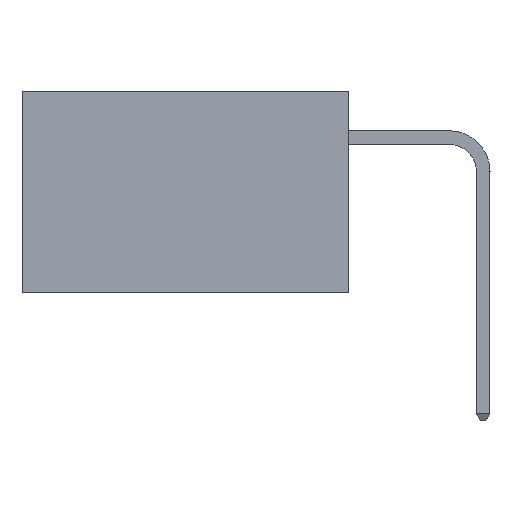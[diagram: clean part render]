
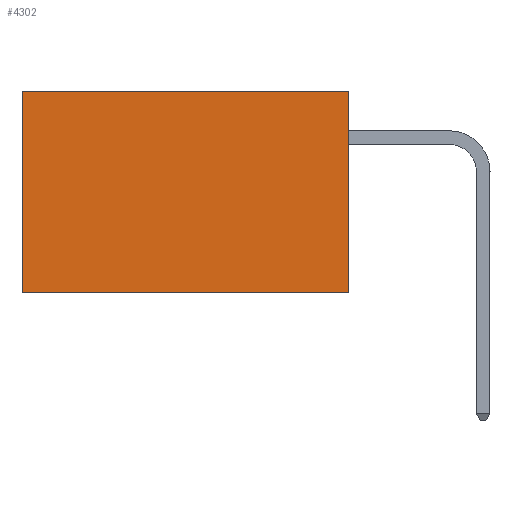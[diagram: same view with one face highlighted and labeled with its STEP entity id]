
A CAD part, left-side view. The second image highlights one B-rep face of the part: STEP entity #4302.
In plain terms, the highlighted planar face has unit normal (-1, 0, 0).
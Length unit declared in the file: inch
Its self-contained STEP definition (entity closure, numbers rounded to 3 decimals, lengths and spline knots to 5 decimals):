
#658 = LINE ( 'NONE', #7100, #45383 ) ;
#1560 = VECTOR ( 'NONE', #34684, 39.37008 ) ;
#1688 = DIRECTION ( 'NONE',  ( 1., 0., 0. ) ) ;
#4302 = ADVANCED_FACE ( 'NONE', ( #34553 ), #45070, .F. ) ;
#4755 = CARTESIAN_POINT ( 'NONE',  ( 0.2875, 0.6, 0. ) ) ;
#6744 = EDGE_CURVE ( 'NONE', #24986, #20230, #19057, .T. ) ;
#7100 = CARTESIAN_POINT ( 'NONE',  ( 0.2875, 0., 0. ) ) ;
#9130 = ORIENTED_EDGE ( 'NONE', *, *, #6744, .F. ) ;
#9705 = EDGE_CURVE ( 'NONE', #24987, #11784, #658, .T. ) ;
#9957 = AXIS2_PLACEMENT_3D ( 'NONE', #23442, #1688, #27096 ) ;
#10304 = CARTESIAN_POINT ( 'NONE',  ( 0.2875, 0., 0. ) ) ;
#11233 = ORIENTED_EDGE ( 'NONE', *, *, #23628, .F. ) ;
#11784 = VERTEX_POINT ( 'NONE', #4755 ) ;
#12401 = LINE ( 'NONE', #31063, #1560 ) ;
#18946 = EDGE_CURVE ( 'NONE', #11784, #20230, #12401, .T. ) ;
#19057 = LINE ( 'NONE', #35641, #46694 ) ;
#19512 = CARTESIAN_POINT ( 'NONE',  ( 0.2875, 0.6, -0.37 ) ) ;
#20230 = VERTEX_POINT ( 'NONE', #19512 ) ;
#23442 = CARTESIAN_POINT ( 'NONE',  ( 0.2875, 0., 0. ) ) ;
#23628 = EDGE_CURVE ( 'NONE', #24987, #24986, #27070, .T. ) ;
#24986 = VERTEX_POINT ( 'NONE', #32379 ) ;
#24987 = VERTEX_POINT ( 'NONE', #25060 ) ;
#25060 = CARTESIAN_POINT ( 'NONE',  ( 0.2875, 0., 0. ) ) ;
#27070 = LINE ( 'NONE', #10304, #35550 ) ;
#27096 = DIRECTION ( 'NONE',  ( 0., 0., -1. ) ) ;
#31063 = CARTESIAN_POINT ( 'NONE',  ( 0.2875, 0.6, 0. ) ) ;
#32379 = CARTESIAN_POINT ( 'NONE',  ( 0.2875, 0., -0.37 ) ) ;
#34553 = FACE_OUTER_BOUND ( 'NONE', #35467, .T. ) ;
#34684 = DIRECTION ( 'NONE',  ( 0., 0., -1. ) ) ;
#35467 = EDGE_LOOP ( 'NONE', ( #45083, #9130, #11233, #43933 ) ) ;
#35550 = VECTOR ( 'NONE', #39427, 39.37008 ) ;
#35641 = CARTESIAN_POINT ( 'NONE',  ( 0.2875, 0., -0.37 ) ) ;
#39427 = DIRECTION ( 'NONE',  ( 0., 0., -1. ) ) ;
#39746 = DIRECTION ( 'NONE',  ( 0., 1., 0. ) ) ;
#43933 = ORIENTED_EDGE ( 'NONE', *, *, #9705, .T. ) ;
#45070 = PLANE ( 'NONE',  #9957 ) ;
#45083 = ORIENTED_EDGE ( 'NONE', *, *, #18946, .T. ) ;
#45383 = VECTOR ( 'NONE', #39746, 39.37008 ) ;
#46283 = DIRECTION ( 'NONE',  ( 0., 1., 0. ) ) ;
#46694 = VECTOR ( 'NONE', #46283, 39.37008 ) ;
